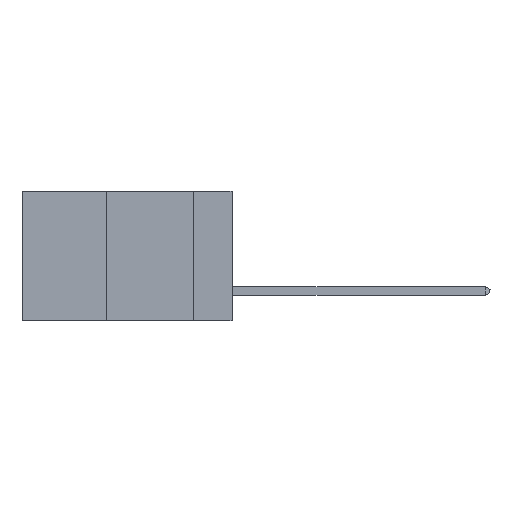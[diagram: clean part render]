
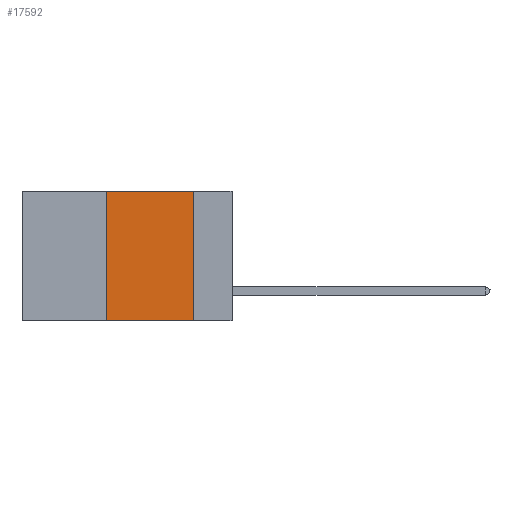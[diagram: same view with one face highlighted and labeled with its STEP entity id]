
A CAD part, left-side view. The second image highlights one B-rep face of the part: STEP entity #17592.
In plain terms, the highlighted planar face has unit normal (-1, 0, 0).
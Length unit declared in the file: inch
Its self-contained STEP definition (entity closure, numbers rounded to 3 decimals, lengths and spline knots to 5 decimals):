
#124 = EDGE_CURVE ( 'NONE', #19831, #34625, #36442, .T. ) ;
#287 = PLANE ( 'NONE',  #15918 ) ;
#6694 = DIRECTION ( 'NONE',  ( 0., -1., 0. ) ) ;
#9008 = CARTESIAN_POINT ( 'NONE',  ( 0., 0.6, 0. ) ) ;
#9402 = CARTESIAN_POINT ( 'NONE',  ( 0., 0.6, -0.37 ) ) ;
#11799 = CARTESIAN_POINT ( 'NONE',  ( 0., 0.36, 0. ) ) ;
#12356 = EDGE_CURVE ( 'NONE', #38262, #34625, #39552, .T. ) ;
#12748 = LINE ( 'NONE', #9008, #25408 ) ;
#14824 = VERTEX_POINT ( 'NONE', #39820 ) ;
#15679 = VECTOR ( 'NONE', #17991, 39.37008 ) ;
#15918 = AXIS2_PLACEMENT_3D ( 'NONE', #18591, #30941, #27955 ) ;
#17592 = ADVANCED_FACE ( 'NONE', ( #40179 ), #287, .F. ) ;
#17991 = DIRECTION ( 'NONE',  ( 0., 0., -1. ) ) ;
#18133 = CARTESIAN_POINT ( 'NONE',  ( 0., 0.11, 0. ) ) ;
#18246 = ORIENTED_EDGE ( 'NONE', *, *, #124, .T. ) ;
#18591 = CARTESIAN_POINT ( 'NONE',  ( 0., 0.6, 0. ) ) ;
#19831 = VERTEX_POINT ( 'NONE', #21784 ) ;
#21784 = CARTESIAN_POINT ( 'NONE',  ( 0., 0.36, -0.37 ) ) ;
#21968 = ORIENTED_EDGE ( 'NONE', *, *, #12356, .F. ) ;
#23562 = EDGE_CURVE ( 'NONE', #14824, #38262, #12748, .T. ) ;
#24574 = EDGE_CURVE ( 'NONE', #19831, #14824, #38509, .T. ) ;
#25408 = VECTOR ( 'NONE', #6694, 39.37008 ) ;
#27955 = DIRECTION ( 'NONE',  ( 0., 0., -1. ) ) ;
#28008 = CARTESIAN_POINT ( 'NONE',  ( 0., 0.11, 0. ) ) ;
#28144 = DIRECTION ( 'NONE',  ( 0., -1., 0. ) ) ;
#30590 = CARTESIAN_POINT ( 'NONE',  ( 0., 0.11, -0.37 ) ) ;
#30941 = DIRECTION ( 'NONE',  ( 1., 0., 0. ) ) ;
#34625 = VERTEX_POINT ( 'NONE', #30590 ) ;
#36220 = ORIENTED_EDGE ( 'NONE', *, *, #24574, .F. ) ;
#36442 = LINE ( 'NONE', #9402, #37878 ) ;
#37014 = DIRECTION ( 'NONE',  ( 0., 0., 1. ) ) ;
#37539 = VECTOR ( 'NONE', #37014, 39.37008 ) ;
#37878 = VECTOR ( 'NONE', #28144, 39.37008 ) ;
#37946 = ORIENTED_EDGE ( 'NONE', *, *, #23562, .F. ) ;
#38262 = VERTEX_POINT ( 'NONE', #28008 ) ;
#38509 = LINE ( 'NONE', #11799, #37539 ) ;
#39552 = LINE ( 'NONE', #18133, #15679 ) ;
#39820 = CARTESIAN_POINT ( 'NONE',  ( 0., 0.36, 0. ) ) ;
#40163 = EDGE_LOOP ( 'NONE', ( #21968, #37946, #36220, #18246 ) ) ;
#40179 = FACE_OUTER_BOUND ( 'NONE', #40163, .T. ) ;
